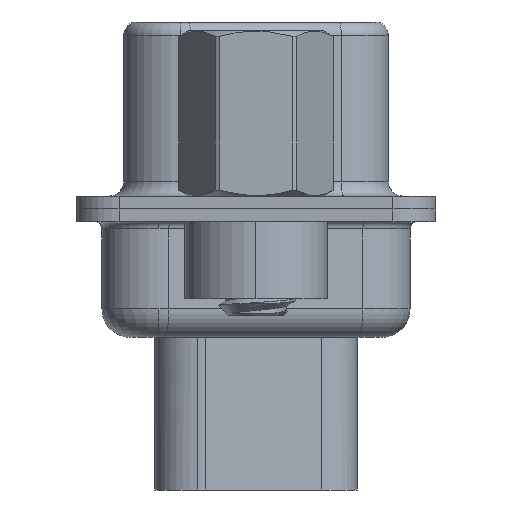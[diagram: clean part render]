
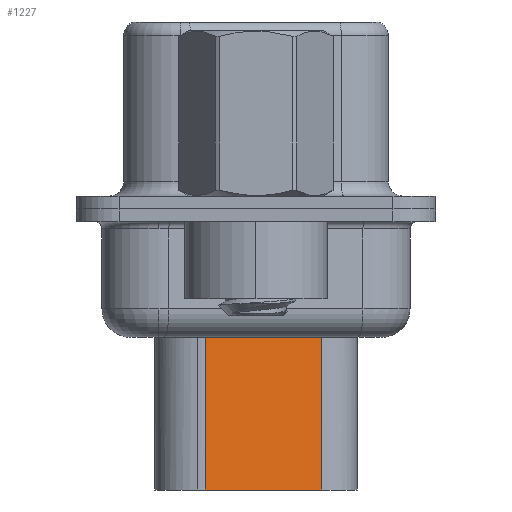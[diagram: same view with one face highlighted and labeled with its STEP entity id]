
A CAD part, left-side view. The second image highlights one B-rep face of the part: STEP entity #1227.
In plain terms, the highlighted planar face has unit normal (-0.985, -0.174, 0).
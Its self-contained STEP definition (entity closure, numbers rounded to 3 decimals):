
#249 = PLANE ( 'NONE',  #676 ) ;
#334 = FACE_OUTER_BOUND ( 'NONE', #5298, .T. ) ;
#676 = AXIS2_PLACEMENT_3D ( 'NONE', #14662, #7408, #3309 ) ;
#845 = CARTESIAN_POINT ( 'NONE',  ( 4.519, 1.78, -9.85 ) ) ;
#938 = LINE ( 'NONE', #845, #10292 ) ;
#1227 = ADVANCED_FACE ( 'NONE', ( #334 ), #249, .T. ) ;
#1551 = CARTESIAN_POINT ( 'NONE',  ( 4.519, 1.78, -9.85 ) ) ;
#2311 = VERTEX_POINT ( 'NONE', #15224 ) ;
#3309 = DIRECTION ( 'NONE',  ( 0.174, -0.985, 0. ) ) ;
#3735 = DIRECTION ( 'NONE',  ( -0.174, 0.985, 0. ) ) ;
#3878 = DIRECTION ( 'NONE',  ( 0., 0., -1. ) ) ;
#4504 = LINE ( 'NONE', #15862, #17593 ) ;
#4914 = ORIENTED_EDGE ( 'NONE', *, *, #13823, .T. ) ;
#5078 = CARTESIAN_POINT ( 'NONE',  ( 5.238, -2.3, -9.85 ) ) ;
#5298 = EDGE_LOOP ( 'NONE', ( #6050, #16662, #4914, #15050 ) ) ;
#5652 = EDGE_CURVE ( 'NONE', #6585, #17777, #938, .T. ) ;
#6050 = ORIENTED_EDGE ( 'NONE', *, *, #9305, .F. ) ;
#6275 = VECTOR ( 'NONE', #10932, 1000. ) ;
#6585 = VERTEX_POINT ( 'NONE', #5078 ) ;
#7408 = DIRECTION ( 'NONE',  ( -0.985, -0.174, 0. ) ) ;
#8167 = LINE ( 'NONE', #16452, #16999 ) ;
#9305 = EDGE_CURVE ( 'NONE', #2311, #6585, #8167, .T. ) ;
#9318 = CARTESIAN_POINT ( 'NONE',  ( 4.519, 1.78, -3.975 ) ) ;
#10022 = EDGE_CURVE ( 'NONE', #2311, #12941, #4504, .T. ) ;
#10099 = DIRECTION ( 'NONE',  ( -0.174, 0.985, 0. ) ) ;
#10292 = VECTOR ( 'NONE', #3735, 1000. ) ;
#10932 = DIRECTION ( 'NONE',  ( 0., 0., -1. ) ) ;
#12316 = CARTESIAN_POINT ( 'NONE',  ( 4.519, 1.78, -3.1 ) ) ;
#12409 = LINE ( 'NONE', #12316, #6275 ) ;
#12941 = VERTEX_POINT ( 'NONE', #9318 ) ;
#13823 = EDGE_CURVE ( 'NONE', #12941, #17777, #12409, .T. ) ;
#14662 = CARTESIAN_POINT ( 'NONE',  ( 4.519, 1.78, -3.1 ) ) ;
#15050 = ORIENTED_EDGE ( 'NONE', *, *, #5652, .F. ) ;
#15224 = CARTESIAN_POINT ( 'NONE',  ( 5.238, -2.3, -3.975 ) ) ;
#15862 = CARTESIAN_POINT ( 'NONE',  ( 4.348, 2.749, -3.975 ) ) ;
#16452 = CARTESIAN_POINT ( 'NONE',  ( 5.238, -2.3, -3.1 ) ) ;
#16662 = ORIENTED_EDGE ( 'NONE', *, *, #10022, .T. ) ;
#16999 = VECTOR ( 'NONE', #3878, 1000. ) ;
#17593 = VECTOR ( 'NONE', #10099, 1000. ) ;
#17777 = VERTEX_POINT ( 'NONE', #1551 ) ;
